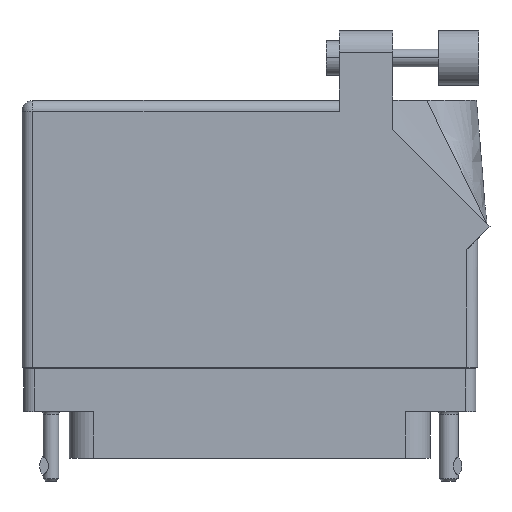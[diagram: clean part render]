
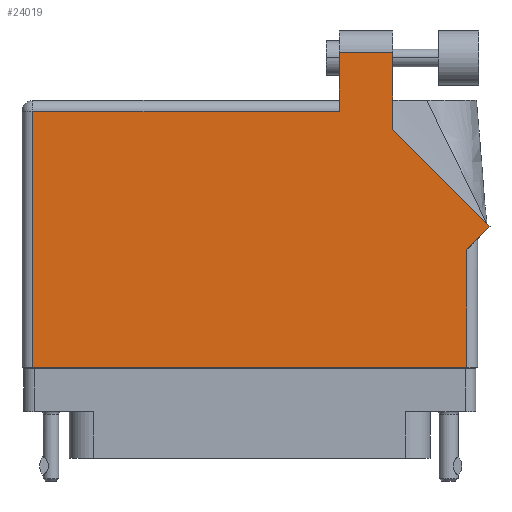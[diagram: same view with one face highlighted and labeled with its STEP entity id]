
A CAD part, front view. The second image highlights one B-rep face of the part: STEP entity #24019.
In plain terms, the highlighted face is planar.
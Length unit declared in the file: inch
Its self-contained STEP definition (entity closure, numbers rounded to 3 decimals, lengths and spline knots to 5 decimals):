
#1670 = VERTEX_POINT ( 'NONE', #27597 ) ;
#1686 = VECTOR ( 'NONE', #32109, 39.37008 ) ;
#1694 = CARTESIAN_POINT ( 'NONE',  ( 0.82, 1.26442, 0.455 ) ) ;
#3012 = EDGE_LOOP ( 'NONE', ( #42115, #56594, #13973, #30680, #59511, #54198, #34699, #60266, #49745 ) ) ;
#4098 = DIRECTION ( 'NONE',  ( -1., 0., 0. ) ) ;
#4231 = CARTESIAN_POINT ( 'NONE',  ( -1.306, 1.43, 0.455 ) ) ;
#5025 = CARTESIAN_POINT ( 'NONE',  ( -1.306, -0.1, 0.455 ) ) ;
#5872 = CARTESIAN_POINT ( 'NONE',  ( -1.244, -0.1, 0.455 ) ) ;
#6097 = VECTOR ( 'NONE', #23548, 39.37008 ) ;
#10998 = LINE ( 'NONE', #14680, #11807 ) ;
#11807 = VECTOR ( 'NONE', #58819, 39.37008 ) ;
#13147 = PLANE ( 'NONE',  #31486 ) ;
#13763 = DIRECTION ( 'NONE',  ( 0., 0., -1. ) ) ;
#13973 = ORIENTED_EDGE ( 'NONE', *, *, #39294, .T. ) ;
#14543 = CARTESIAN_POINT ( 'NONE',  ( 1.244, -0.1, 0.455 ) ) ;
#14574 = DIRECTION ( 'NONE',  ( -1., 0., 0. ) ) ;
#14680 = CARTESIAN_POINT ( 'NONE',  ( 0.513, 1.43, 0.455 ) ) ;
#15900 = VECTOR ( 'NONE', #38707, 39.37008 ) ;
#16264 = EDGE_CURVE ( 'NONE', #37604, #22785, #34943, .T. ) ;
#16602 = EDGE_CURVE ( 'NONE', #1670, #41861, #31949, .T. ) ;
#18461 = CARTESIAN_POINT ( 'NONE',  ( 1.244, 0.637, 0.455 ) ) ;
#18629 = CARTESIAN_POINT ( 'NONE',  ( 1.37671, 0.70771, 0.455 ) ) ;
#22452 = DIRECTION ( 'NONE',  ( 0.707, 0.707, 0. ) ) ;
#22785 = VERTEX_POINT ( 'NONE', #32475 ) ;
#23133 = CARTESIAN_POINT ( 'NONE',  ( 0.513, 1.705, 0.455 ) ) ;
#23548 = DIRECTION ( 'NONE',  ( -1., 0., 0. ) ) ;
#24019 = ADVANCED_FACE ( 'NONE', ( #37588 ), #13147, .F. ) ;
#24833 = LINE ( 'NONE', #27624, #38882 ) ;
#25478 = CARTESIAN_POINT ( 'NONE',  ( 0.513, 1.705, 0.455 ) ) ;
#26481 = VECTOR ( 'NONE', #50922, 39.37008 ) ;
#27597 = CARTESIAN_POINT ( 'NONE',  ( 0.82, 1.705, 0.455 ) ) ;
#27624 = CARTESIAN_POINT ( 'NONE',  ( -1.306, 1.368, 0.455 ) ) ;
#30680 = ORIENTED_EDGE ( 'NONE', *, *, #51712, .T. ) ;
#30965 = CARTESIAN_POINT ( 'NONE',  ( 1.37671, 0.70771, 0.455 ) ) ;
#31486 = AXIS2_PLACEMENT_3D ( 'NONE', #4231, #13763, #14574 ) ;
#31949 = LINE ( 'NONE', #23133, #6097 ) ;
#32109 = DIRECTION ( 'NONE',  ( 0., 1., 0. ) ) ;
#32475 = CARTESIAN_POINT ( 'NONE',  ( 1.244, 0.575, 0.455 ) ) ;
#32701 = LINE ( 'NONE', #38226, #34934 ) ;
#33725 = VECTOR ( 'NONE', #43181, 39.37008 ) ;
#34699 = ORIENTED_EDGE ( 'NONE', *, *, #16264, .T. ) ;
#34934 = VECTOR ( 'NONE', #47645, 39.37008 ) ;
#34943 = LINE ( 'NONE', #18461, #1686 ) ;
#35674 = VERTEX_POINT ( 'NONE', #38987 ) ;
#37116 = CARTESIAN_POINT ( 'NONE',  ( 1.306, 0.637, 0.455 ) ) ;
#37588 = FACE_OUTER_BOUND ( 'NONE', #3012, .T. ) ;
#37604 = VERTEX_POINT ( 'NONE', #14543 ) ;
#38226 = CARTESIAN_POINT ( 'NONE',  ( 0.82, 1.26442, 0.455 ) ) ;
#38707 = DIRECTION ( 'NONE',  ( 0., -1., 0. ) ) ;
#38882 = VECTOR ( 'NONE', #4098, 39.37008 ) ;
#38987 = CARTESIAN_POINT ( 'NONE',  ( 0.513, 1.368, 0.455 ) ) ;
#39294 = EDGE_CURVE ( 'NONE', #41861, #35674, #10998, .T. ) ;
#41861 = VERTEX_POINT ( 'NONE', #25478 ) ;
#42115 = ORIENTED_EDGE ( 'NONE', *, *, #54249, .T. ) ;
#42245 = VERTEX_POINT ( 'NONE', #18629 ) ;
#42487 = LINE ( 'NONE', #5872, #15900 ) ;
#42656 = EDGE_CURVE ( 'NONE', #56349, #37604, #46228, .T. ) ;
#43181 = DIRECTION ( 'NONE',  ( 1., 0., 0. ) ) ;
#43961 = CARTESIAN_POINT ( 'NONE',  ( -1.244, -0.1, 0.455 ) ) ;
#45468 = VECTOR ( 'NONE', #22452, 39.37008 ) ;
#46228 = LINE ( 'NONE', #5025, #33725 ) ;
#47645 = DIRECTION ( 'NONE',  ( 0., 1., 0. ) ) ;
#48479 = CARTESIAN_POINT ( 'NONE',  ( -1.244, 1.368, 0.455 ) ) ;
#49699 = VERTEX_POINT ( 'NONE', #1694 ) ;
#49745 = ORIENTED_EDGE ( 'NONE', *, *, #58796, .T. ) ;
#50439 = VERTEX_POINT ( 'NONE', #48479 ) ;
#50922 = DIRECTION ( 'NONE',  ( -0.707, 0.707, 0. ) ) ;
#51712 = EDGE_CURVE ( 'NONE', #35674, #50439, #24833, .T. ) ;
#51757 = EDGE_CURVE ( 'NONE', #22785, #42245, #59445, .T. ) ;
#54198 = ORIENTED_EDGE ( 'NONE', *, *, #42656, .T. ) ;
#54249 = EDGE_CURVE ( 'NONE', #49699, #1670, #32701, .T. ) ;
#56349 = VERTEX_POINT ( 'NONE', #43961 ) ;
#56594 = ORIENTED_EDGE ( 'NONE', *, *, #16602, .T. ) ;
#58796 = EDGE_CURVE ( 'NONE', #42245, #49699, #58905, .T. ) ;
#58819 = DIRECTION ( 'NONE',  ( 0., -1., 0. ) ) ;
#58905 = LINE ( 'NONE', #30965, #26481 ) ;
#59445 = LINE ( 'NONE', #37116, #45468 ) ;
#59511 = ORIENTED_EDGE ( 'NONE', *, *, #61024, .T. ) ;
#60266 = ORIENTED_EDGE ( 'NONE', *, *, #51757, .T. ) ;
#61024 = EDGE_CURVE ( 'NONE', #50439, #56349, #42487, .T. ) ;
